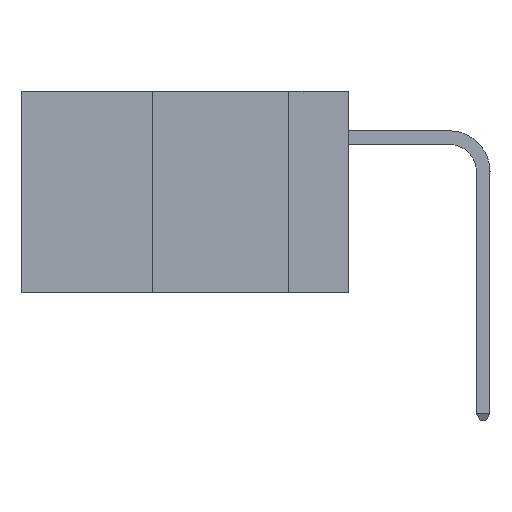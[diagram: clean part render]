
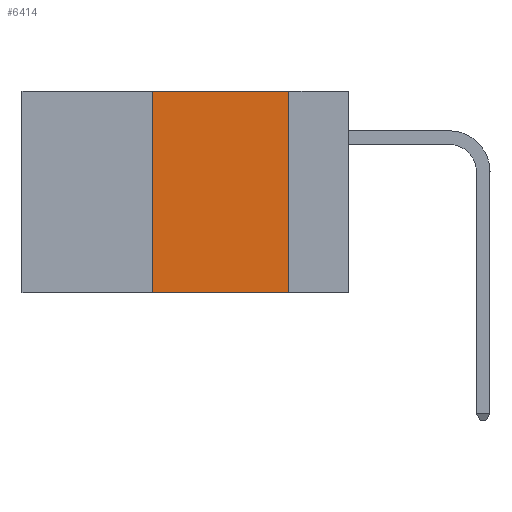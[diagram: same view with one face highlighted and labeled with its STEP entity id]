
A CAD part, left-side view. The second image highlights one B-rep face of the part: STEP entity #6414.
In plain terms, the highlighted planar face has unit normal (-1, 0, 0).
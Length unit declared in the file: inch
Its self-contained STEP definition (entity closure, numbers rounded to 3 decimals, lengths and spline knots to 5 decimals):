
#671 = ORIENTED_EDGE ( 'NONE', *, *, #21664, .F. ) ;
#4719 = CARTESIAN_POINT ( 'NONE',  ( 0., 0.6, 0. ) ) ;
#4786 = EDGE_LOOP ( 'NONE', ( #5600, #671, #34154, #9177 ) ) ;
#5600 = ORIENTED_EDGE ( 'NONE', *, *, #31260, .F. ) ;
#6414 = ADVANCED_FACE ( 'NONE', ( #34373 ), #25126, .F. ) ;
#7850 = LINE ( 'NONE', #4719, #10847 ) ;
#8272 = VERTEX_POINT ( 'NONE', #10419 ) ;
#9177 = ORIENTED_EDGE ( 'NONE', *, *, #41451, .T. ) ;
#9803 = LINE ( 'NONE', #11392, #46993 ) ;
#10419 = CARTESIAN_POINT ( 'NONE',  ( 0., 0.36, -0.37 ) ) ;
#10443 = CARTESIAN_POINT ( 'NONE',  ( 0., 0.6, 0. ) ) ;
#10847 = VECTOR ( 'NONE', #46854, 39.37008 ) ;
#11392 = CARTESIAN_POINT ( 'NONE',  ( 0., 0.36, 0. ) ) ;
#12341 = CARTESIAN_POINT ( 'NONE',  ( 0., 0.11, 0. ) ) ;
#13628 = LINE ( 'NONE', #35649, #24374 ) ;
#15486 = VECTOR ( 'NONE', #31420, 39.37008 ) ;
#17423 = VERTEX_POINT ( 'NONE', #23351 ) ;
#21664 = EDGE_CURVE ( 'NONE', #17423, #46451, #7850, .T. ) ;
#23351 = CARTESIAN_POINT ( 'NONE',  ( 0., 0.36, 0. ) ) ;
#24374 = VECTOR ( 'NONE', #35968, 39.37008 ) ;
#25007 = CARTESIAN_POINT ( 'NONE',  ( 0., 0.11, -0.37 ) ) ;
#25126 = PLANE ( 'NONE',  #25194 ) ;
#25194 = AXIS2_PLACEMENT_3D ( 'NONE', #10443, #41185, #41352 ) ;
#27550 = VERTEX_POINT ( 'NONE', #25007 ) ;
#28712 = LINE ( 'NONE', #43205, #15486 ) ;
#31260 = EDGE_CURVE ( 'NONE', #46451, #27550, #28712, .T. ) ;
#31420 = DIRECTION ( 'NONE',  ( 0., 0., -1. ) ) ;
#34154 = ORIENTED_EDGE ( 'NONE', *, *, #37536, .F. ) ;
#34373 = FACE_OUTER_BOUND ( 'NONE', #4786, .T. ) ;
#34896 = DIRECTION ( 'NONE',  ( 0., 0., 1. ) ) ;
#35649 = CARTESIAN_POINT ( 'NONE',  ( 0., 0.6, -0.37 ) ) ;
#35968 = DIRECTION ( 'NONE',  ( 0., -1., 0. ) ) ;
#37536 = EDGE_CURVE ( 'NONE', #8272, #17423, #9803, .T. ) ;
#41185 = DIRECTION ( 'NONE',  ( 1., 0., 0. ) ) ;
#41352 = DIRECTION ( 'NONE',  ( 0., 0., -1. ) ) ;
#41451 = EDGE_CURVE ( 'NONE', #8272, #27550, #13628, .T. ) ;
#43205 = CARTESIAN_POINT ( 'NONE',  ( 0., 0.11, 0. ) ) ;
#46451 = VERTEX_POINT ( 'NONE', #12341 ) ;
#46854 = DIRECTION ( 'NONE',  ( 0., -1., 0. ) ) ;
#46993 = VECTOR ( 'NONE', #34896, 39.37008 ) ;
